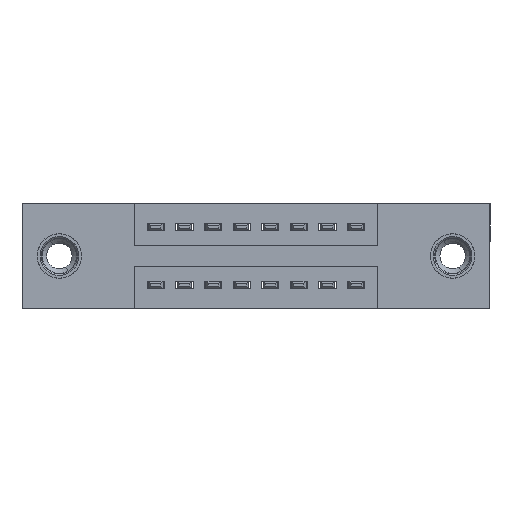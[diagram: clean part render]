
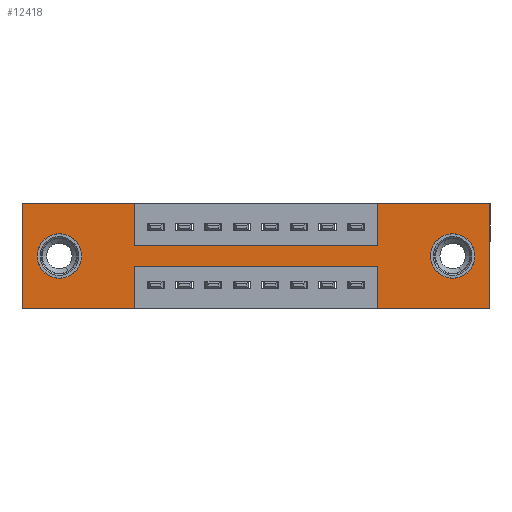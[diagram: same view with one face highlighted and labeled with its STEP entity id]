
A CAD part, front view. The second image highlights one B-rep face of the part: STEP entity #12418.
In plain terms, the highlighted planar face has unit normal (0, -1, 0).
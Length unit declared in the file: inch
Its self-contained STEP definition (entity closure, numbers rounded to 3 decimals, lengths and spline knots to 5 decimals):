
#26 = LINE ( 'NONE', #3558, #6138 ) ;
#39 = FACE_OUTER_BOUND ( 'NONE', #14598, .T. ) ;
#166 = LINE ( 'NONE', #2154, #9826 ) ;
#249 = VECTOR ( 'NONE', #14134, 39.37008 ) ;
#258 = DIRECTION ( 'NONE',  ( 0., 0., -1. ) ) ;
#369 = EDGE_CURVE ( 'NONE', #889, #7056, #970, .T. ) ;
#821 = VECTOR ( 'NONE', #6390, 39.37008 ) ;
#874 = ORIENTED_EDGE ( 'NONE', *, *, #13661, .T. ) ;
#889 = VERTEX_POINT ( 'NONE', #5376 ) ;
#970 = LINE ( 'NONE', #3398, #14050 ) ;
#985 = VERTEX_POINT ( 'NONE', #8876 ) ;
#1015 = DIRECTION ( 'NONE',  ( 0., 0., -1. ) ) ;
#1043 = ORIENTED_EDGE ( 'NONE', *, *, #12865, .F. ) ;
#1198 = CARTESIAN_POINT ( 'NONE',  ( 0.3925, 0., -0.37 ) ) ;
#1239 = EDGE_CURVE ( 'NONE', #3006, #10958, #7289, .T. ) ;
#1459 = ORIENTED_EDGE ( 'NONE', *, *, #12045, .F. ) ;
#1482 = AXIS2_PLACEMENT_3D ( 'NONE', #8156, #8268, #1015 ) ;
#1594 = ORIENTED_EDGE ( 'NONE', *, *, #1777, .F. ) ;
#1720 = ORIENTED_EDGE ( 'NONE', *, *, #10818, .T. ) ;
#1777 = EDGE_CURVE ( 'NONE', #1969, #3929, #13379, .T. ) ;
#1816 = LINE ( 'NONE', #7185, #14089 ) ;
#1858 = EDGE_LOOP ( 'NONE', ( #874, #2793 ) ) ;
#1964 = CARTESIAN_POINT ( 'NONE',  ( 0., 0., 0. ) ) ;
#1969 = VERTEX_POINT ( 'NONE', #13717 ) ;
#2154 = CARTESIAN_POINT ( 'NONE',  ( 1.635, 0., 0. ) ) ;
#2551 = LINE ( 'NONE', #11855, #5015 ) ;
#2705 = ORIENTED_EDGE ( 'NONE', *, *, #11641, .F. ) ;
#2793 = ORIENTED_EDGE ( 'NONE', *, *, #4115, .T. ) ;
#2799 = ORIENTED_EDGE ( 'NONE', *, *, #4786, .F. ) ;
#3006 = VERTEX_POINT ( 'NONE', #11074 ) ;
#3018 = EDGE_CURVE ( 'NONE', #10958, #13876, #10410, .T. ) ;
#3038 = ORIENTED_EDGE ( 'NONE', *, *, #4805, .F. ) ;
#3092 = VECTOR ( 'NONE', #5805, 39.37008 ) ;
#3303 = CARTESIAN_POINT ( 'NONE',  ( 1.2425, 0., -0.15 ) ) ;
#3331 = VERTEX_POINT ( 'NONE', #5617 ) ;
#3353 = FACE_BOUND ( 'NONE', #6670, .T. ) ;
#3398 = CARTESIAN_POINT ( 'NONE',  ( 0.3925, 0., -0.22 ) ) ;
#3440 = ORIENTED_EDGE ( 'NONE', *, *, #1239, .F. ) ;
#3558 = CARTESIAN_POINT ( 'NONE',  ( 0., 0., 0. ) ) ;
#3632 = DIRECTION ( 'NONE',  ( -1., 0., 0. ) ) ;
#3712 = EDGE_CURVE ( 'NONE', #13876, #7758, #2551, .T. ) ;
#3876 = VERTEX_POINT ( 'NONE', #10439 ) ;
#3893 = VERTEX_POINT ( 'NONE', #1198 ) ;
#3929 = VERTEX_POINT ( 'NONE', #1964 ) ;
#4115 = EDGE_CURVE ( 'NONE', #15208, #10259, #4451, .T. ) ;
#4345 = CARTESIAN_POINT ( 'NONE',  ( 0., 0., -0.37 ) ) ;
#4443 = EDGE_CURVE ( 'NONE', #13699, #889, #14208, .T. ) ;
#4451 = CIRCLE ( 'NONE', #4833, 0.078 ) ;
#4629 = ORIENTED_EDGE ( 'NONE', *, *, #4443, .F. ) ;
#4687 = CARTESIAN_POINT ( 'NONE',  ( 0.13, 0., -0.185 ) ) ;
#4781 = DIRECTION ( 'NONE',  ( 1., 0., 0. ) ) ;
#4786 = EDGE_CURVE ( 'NONE', #3876, #985, #166, .T. ) ;
#4805 = EDGE_CURVE ( 'NONE', #3929, #3006, #15272, .T. ) ;
#4833 = AXIS2_PLACEMENT_3D ( 'NONE', #11322, #11372, #11254 ) ;
#5015 = VECTOR ( 'NONE', #11839, 39.37008 ) ;
#5127 = CARTESIAN_POINT ( 'NONE',  ( 0., 0., -0.37 ) ) ;
#5178 = VECTOR ( 'NONE', #6382, 39.37008 ) ;
#5376 = CARTESIAN_POINT ( 'NONE',  ( 1.2425, 0., -0.22 ) ) ;
#5533 = DIRECTION ( 'NONE',  ( -1., 0., 0. ) ) ;
#5617 = CARTESIAN_POINT ( 'NONE',  ( 0.13, 0., -0.263 ) ) ;
#5805 = DIRECTION ( 'NONE',  ( 1., 0., 0. ) ) ;
#5809 = CARTESIAN_POINT ( 'NONE',  ( 1.2425, 0., 0. ) ) ;
#5851 = CARTESIAN_POINT ( 'NONE',  ( 1.505, 0., -0.263 ) ) ;
#5867 = DIRECTION ( 'NONE',  ( 0., 0., 1. ) ) ;
#5930 = CIRCLE ( 'NONE', #14933, 0.078 ) ;
#6120 = ORIENTED_EDGE ( 'NONE', *, *, #369, .F. ) ;
#6136 = CARTESIAN_POINT ( 'NONE',  ( 0.13, 0., -0.185 ) ) ;
#6138 = VECTOR ( 'NONE', #4781, 39.37008 ) ;
#6382 = DIRECTION ( 'NONE',  ( 0., 0., 1. ) ) ;
#6390 = DIRECTION ( 'NONE',  ( 0., 0., -1. ) ) ;
#6509 = CARTESIAN_POINT ( 'NONE',  ( 0., 0., 0. ) ) ;
#6670 = EDGE_LOOP ( 'NONE', ( #10773, #1720 ) ) ;
#7041 = CARTESIAN_POINT ( 'NONE',  ( 0.13, 0., -0.107 ) ) ;
#7056 = VERTEX_POINT ( 'NONE', #8025 ) ;
#7057 = CIRCLE ( 'NONE', #7070, 0.078 ) ;
#7070 = AXIS2_PLACEMENT_3D ( 'NONE', #6136, #14371, #7342 ) ;
#7073 = PLANE ( 'NONE',  #1482 ) ;
#7185 = CARTESIAN_POINT ( 'NONE',  ( 0.3925, 0., -0.37 ) ) ;
#7264 = VECTOR ( 'NONE', #8485, 39.37008 ) ;
#7289 = LINE ( 'NONE', #7682, #821 ) ;
#7342 = DIRECTION ( 'NONE',  ( 0., 0., 1. ) ) ;
#7484 = LINE ( 'NONE', #5127, #13016 ) ;
#7536 = DIRECTION ( 'NONE',  ( 0., 1., 0. ) ) ;
#7682 = CARTESIAN_POINT ( 'NONE',  ( 0.3925, 0., 0. ) ) ;
#7758 = VERTEX_POINT ( 'NONE', #5809 ) ;
#7841 = ORIENTED_EDGE ( 'NONE', *, *, #3712, .F. ) ;
#8025 = CARTESIAN_POINT ( 'NONE',  ( 0.3925, 0., -0.22 ) ) ;
#8156 = CARTESIAN_POINT ( 'NONE',  ( 0., 0., -0.37 ) ) ;
#8268 = DIRECTION ( 'NONE',  ( 0., -1., 0. ) ) ;
#8360 = VERTEX_POINT ( 'NONE', #7041 ) ;
#8485 = DIRECTION ( 'NONE',  ( 1., 0., 0. ) ) ;
#8876 = CARTESIAN_POINT ( 'NONE',  ( 1.635, 0., -0.37 ) ) ;
#9331 = CARTESIAN_POINT ( 'NONE',  ( 1.505, 0., -0.107 ) ) ;
#9409 = LINE ( 'NONE', #4345, #12147 ) ;
#9544 = CARTESIAN_POINT ( 'NONE',  ( 0.3925, 0., -0.15 ) ) ;
#9707 = FACE_BOUND ( 'NONE', #1858, .T. ) ;
#9826 = VECTOR ( 'NONE', #11655, 39.37008 ) ;
#10259 = VERTEX_POINT ( 'NONE', #9331 ) ;
#10410 = LINE ( 'NONE', #9544, #7264 ) ;
#10439 = CARTESIAN_POINT ( 'NONE',  ( 1.635, 0., 0. ) ) ;
#10773 = ORIENTED_EDGE ( 'NONE', *, *, #13572, .T. ) ;
#10818 = EDGE_CURVE ( 'NONE', #3331, #8360, #11209, .T. ) ;
#10958 = VERTEX_POINT ( 'NONE', #14312 ) ;
#11074 = CARTESIAN_POINT ( 'NONE',  ( 0.3925, 0., 0. ) ) ;
#11209 = CIRCLE ( 'NONE', #12882, 0.078 ) ;
#11254 = DIRECTION ( 'NONE',  ( 0., 0., -1. ) ) ;
#11322 = CARTESIAN_POINT ( 'NONE',  ( 1.505, 0., -0.185 ) ) ;
#11372 = DIRECTION ( 'NONE',  ( 0., 1., 0. ) ) ;
#11641 = EDGE_CURVE ( 'NONE', #985, #13699, #7484, .T. ) ;
#11655 = DIRECTION ( 'NONE',  ( 0., 0., -1. ) ) ;
#11839 = DIRECTION ( 'NONE',  ( 0., 0., 1. ) ) ;
#11855 = CARTESIAN_POINT ( 'NONE',  ( 1.2425, 0., 0. ) ) ;
#12045 = EDGE_CURVE ( 'NONE', #7056, #3893, #1816, .T. ) ;
#12147 = VECTOR ( 'NONE', #5533, 39.37008 ) ;
#12281 = CARTESIAN_POINT ( 'NONE',  ( 1.2425, 0., -0.37 ) ) ;
#12418 = ADVANCED_FACE ( 'NONE', ( #9707, #3353, #39 ), #7073, .T. ) ;
#12865 = EDGE_CURVE ( 'NONE', #7758, #3876, #26, .T. ) ;
#12882 = AXIS2_PLACEMENT_3D ( 'NONE', #4687, #12946, #5867 ) ;
#12946 = DIRECTION ( 'NONE',  ( 0., 1., 0. ) ) ;
#13016 = VECTOR ( 'NONE', #13331, 39.37008 ) ;
#13331 = DIRECTION ( 'NONE',  ( -1., 0., 0. ) ) ;
#13379 = LINE ( 'NONE', #6509, #249 ) ;
#13457 = CARTESIAN_POINT ( 'NONE',  ( 1.2425, 0., -0.37 ) ) ;
#13572 = EDGE_CURVE ( 'NONE', #8360, #3331, #7057, .T. ) ;
#13661 = EDGE_CURVE ( 'NONE', #10259, #15208, #5930, .T. ) ;
#13699 = VERTEX_POINT ( 'NONE', #12281 ) ;
#13717 = CARTESIAN_POINT ( 'NONE',  ( 0., 0., -0.37 ) ) ;
#13876 = VERTEX_POINT ( 'NONE', #3303 ) ;
#14047 = CARTESIAN_POINT ( 'NONE',  ( 0., 0., 0. ) ) ;
#14050 = VECTOR ( 'NONE', #3632, 39.37008 ) ;
#14089 = VECTOR ( 'NONE', #15379, 39.37008 ) ;
#14134 = DIRECTION ( 'NONE',  ( 0., 0., 1. ) ) ;
#14208 = LINE ( 'NONE', #13457, #5178 ) ;
#14312 = CARTESIAN_POINT ( 'NONE',  ( 0.3925, 0., -0.15 ) ) ;
#14371 = DIRECTION ( 'NONE',  ( 0., 1., 0. ) ) ;
#14380 = ORIENTED_EDGE ( 'NONE', *, *, #14775, .F. ) ;
#14562 = CARTESIAN_POINT ( 'NONE',  ( 1.505, 0., -0.185 ) ) ;
#14598 = EDGE_LOOP ( 'NONE', ( #1459, #6120, #4629, #2705, #2799, #1043, #7841, #14896, #3440, #3038, #1594, #14380 ) ) ;
#14775 = EDGE_CURVE ( 'NONE', #3893, #1969, #9409, .T. ) ;
#14896 = ORIENTED_EDGE ( 'NONE', *, *, #3018, .F. ) ;
#14933 = AXIS2_PLACEMENT_3D ( 'NONE', #14562, #7536, #258 ) ;
#15208 = VERTEX_POINT ( 'NONE', #5851 ) ;
#15272 = LINE ( 'NONE', #14047, #3092 ) ;
#15379 = DIRECTION ( 'NONE',  ( 0., 0., -1. ) ) ;
